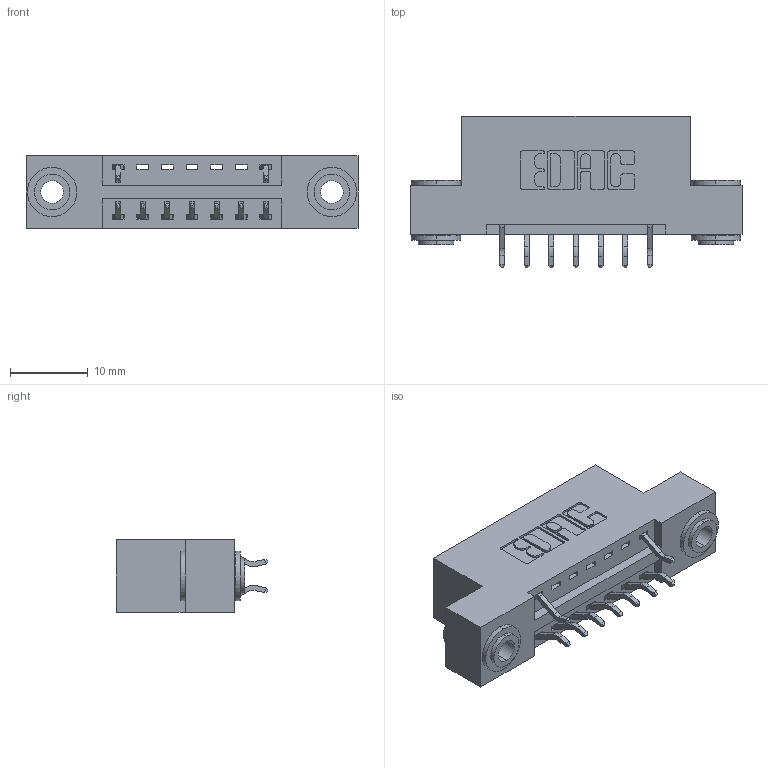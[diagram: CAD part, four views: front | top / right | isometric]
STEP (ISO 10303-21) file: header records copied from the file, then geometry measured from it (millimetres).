
FILE_DESCRIPTION (( 'STEP AP203' ), '1' );
FILE_NAME ('346-014-556-203.STEP', '2018-08-20T01:43:34', ( '' ), ( '' ), 'SwSTEP 2.0', 'SolidWorks 2016', '' );
FILE_SCHEMA (( 'CONFIG_CONTROL_DESIGN' ));
Length unit declared in the file: inch
Products named in the file (4): 345-250-002_345-250-002-102; 346-014-556-203; 345-292-001_556 Tail; 346 Part_Flush Mounting Lugs - 0.156 Dia-TH
Assembly tree (12 placements, depth 2):
  346-014-556-203
    346 Part_Flush Mounting Lugs - 0.156 Dia-TH
    345-292-001_556 Tail  x9
    345-250-002_345-250-002-102  x2
Bounding box: 42.8 x 19.57 x 9.4 mm (x, y, z)
Volume: 3875.6 mm3; surface area: 4723.6 mm2
Topology: 12 solids, 12 shells, 712 faces, 2067 edges, 1362 vertices
Faces by surface type: plane 462, cylinder 242, cone 8
Entity records: 9990 total; most frequent: CARTESIAN_POINT 1706, ORIENTED_EDGE 1626, DIRECTION 1569, EDGE_CURVE 813, VECTOR 621, LINE 621, VERTEX_POINT 538, AXIS2_PLACEMENT_3D 474
